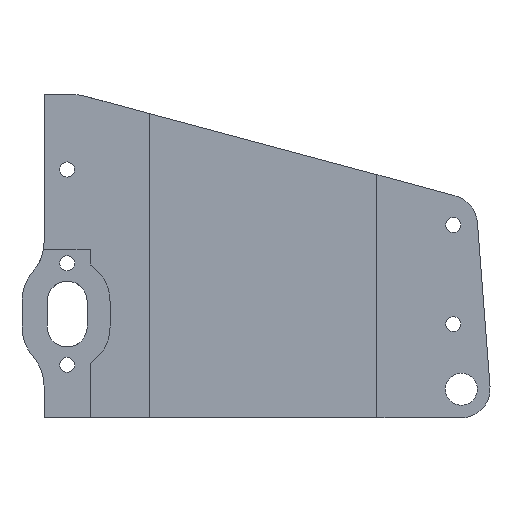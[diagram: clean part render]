
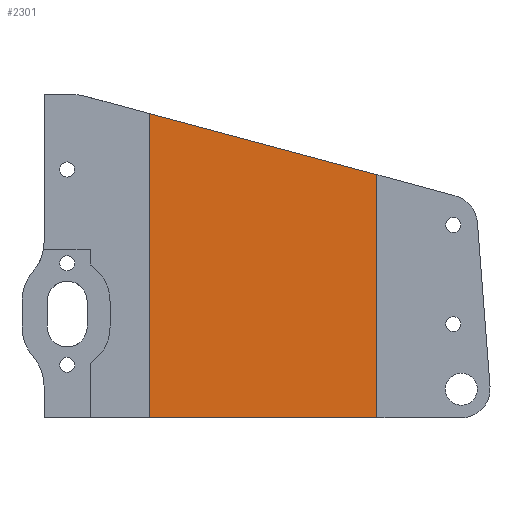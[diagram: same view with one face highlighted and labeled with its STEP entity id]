
A CAD part, front view. The second image highlights one B-rep face of the part: STEP entity #2301.
In plain terms, the highlighted planar face has unit normal (0, -1, 0).
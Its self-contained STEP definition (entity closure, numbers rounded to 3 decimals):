
#48 = DIRECTION ( 'NONE',  ( 0., 0., 1. ) ) ;
#154 = CARTESIAN_POINT ( 'NONE',  ( 21.006, 0.457, -3.879 ) ) ;
#182 = EDGE_CURVE ( 'NONE', #824, #487, #1782, .T. ) ;
#183 = CARTESIAN_POINT ( 'NONE',  ( 0., 0.457, 0. ) ) ;
#191 = DIRECTION ( 'NONE',  ( 0., 0., 1. ) ) ;
#315 = CARTESIAN_POINT ( 'NONE',  ( 0., 0.457, -64.364 ) ) ;
#382 = DIRECTION ( 'NONE',  ( 0., 0., 1. ) ) ;
#487 = VERTEX_POINT ( 'NONE', #154 ) ;
#583 = VECTOR ( 'NONE', #48, 1000. ) ;
#666 = VECTOR ( 'NONE', #2642, 1000. ) ;
#687 = EDGE_CURVE ( 'NONE', #1316, #824, #2243, .T. ) ;
#824 = VERTEX_POINT ( 'NONE', #1931 ) ;
#882 = VECTOR ( 'NONE', #1776, 1000. ) ;
#1042 = ORIENTED_EDGE ( 'NONE', *, *, #1203, .F. ) ;
#1119 = VECTOR ( 'NONE', #382, 1000. ) ;
#1175 = ORIENTED_EDGE ( 'NONE', *, *, #1870, .T. ) ;
#1194 = LINE ( 'NONE', #1824, #1119 ) ;
#1203 = EDGE_CURVE ( 'NONE', #2319, #487, #1194, .T. ) ;
#1224 = CARTESIAN_POINT ( 'NONE',  ( 21.006, 0.457, -64.364 ) ) ;
#1316 = VERTEX_POINT ( 'NONE', #1672 ) ;
#1375 = FACE_OUTER_BOUND ( 'NONE', #2416, .T. ) ;
#1396 = CARTESIAN_POINT ( 'NONE',  ( 0.444, 0.457, 1.65 ) ) ;
#1422 = DIRECTION ( 'NONE',  ( 0., 1., 0. ) ) ;
#1436 = LINE ( 'NONE', #315, #882 ) ;
#1509 = ORIENTED_EDGE ( 'NONE', *, *, #687, .T. ) ;
#1672 = CARTESIAN_POINT ( 'NONE',  ( 66.167, 0.457, -64.364 ) ) ;
#1776 = DIRECTION ( 'NONE',  ( 1., 0., 0. ) ) ;
#1782 = LINE ( 'NONE', #1396, #666 ) ;
#1813 = AXIS2_PLACEMENT_3D ( 'NONE', #183, #1422, #191 ) ;
#1824 = CARTESIAN_POINT ( 'NONE',  ( 21.006, 0.457, 0. ) ) ;
#1870 = EDGE_CURVE ( 'NONE', #2319, #1316, #1436, .T. ) ;
#1931 = CARTESIAN_POINT ( 'NONE',  ( 66.167, 0.457, -16.023 ) ) ;
#2105 = CARTESIAN_POINT ( 'NONE',  ( 66.167, 0.457, 0. ) ) ;
#2243 = LINE ( 'NONE', #2105, #583 ) ;
#2262 = PLANE ( 'NONE',  #1813 ) ;
#2301 = ADVANCED_FACE ( 'NONE', ( #1375 ), #2262, .F. ) ;
#2319 = VERTEX_POINT ( 'NONE', #1224 ) ;
#2416 = EDGE_LOOP ( 'NONE', ( #1509, #2520, #1042, #1175 ) ) ;
#2520 = ORIENTED_EDGE ( 'NONE', *, *, #182, .T. ) ;
#2642 = DIRECTION ( 'NONE',  ( -0.966, 0., 0.26 ) ) ;
